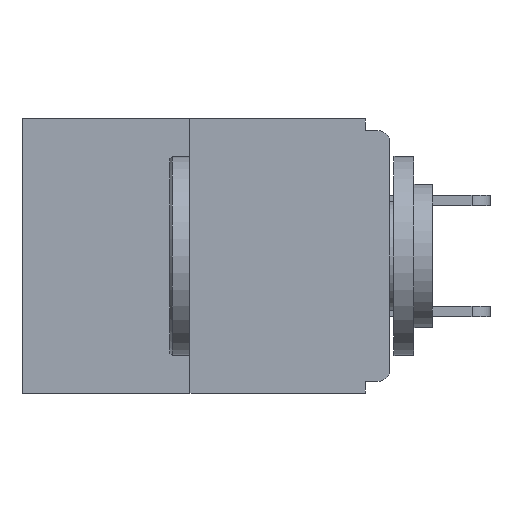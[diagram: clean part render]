
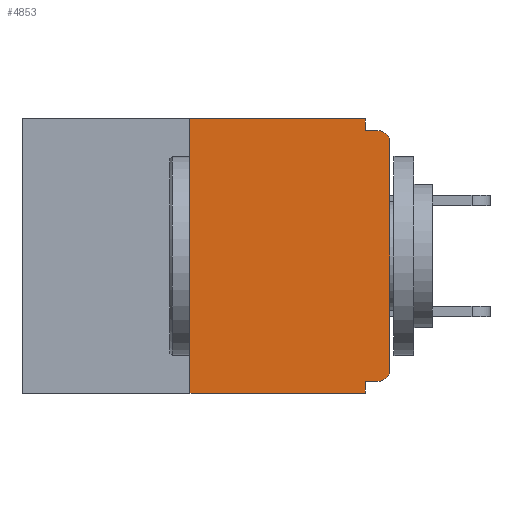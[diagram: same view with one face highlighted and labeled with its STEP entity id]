
A CAD part, left-side view. The second image highlights one B-rep face of the part: STEP entity #4853.
In plain terms, the highlighted planar face has unit normal (-1, 0, 0).
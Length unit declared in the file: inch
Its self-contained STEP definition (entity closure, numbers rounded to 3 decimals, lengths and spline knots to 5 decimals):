
#928 = CARTESIAN_POINT ( 'NONE',  ( 0., 0., -0.03 ) ) ;
#980 = DIRECTION ( 'NONE',  ( 0., 0., -1. ) ) ;
#1677 = VERTEX_POINT ( 'NONE', #18223 ) ;
#1706 = CARTESIAN_POINT ( 'NONE',  ( 0., 0., -0.328 ) ) ;
#1978 = CARTESIAN_POINT ( 'NONE',  ( 0., 0.031, -0.343 ) ) ;
#2062 = EDGE_CURVE ( 'NONE', #12273, #8762, #14587, .T. ) ;
#2663 = CARTESIAN_POINT ( 'NONE',  ( 0., 0.25, -0.343 ) ) ;
#2809 = EDGE_CURVE ( 'NONE', #20549, #18197, #7778, .T. ) ;
#2960 = DIRECTION ( 'NONE',  ( 1., 0., 0. ) ) ;
#3241 = ORIENTED_EDGE ( 'NONE', *, *, #2062, .T. ) ;
#3322 = VECTOR ( 'NONE', #9281, 39.37008 ) ;
#3625 = ORIENTED_EDGE ( 'NONE', *, *, #2809, .F. ) ;
#3954 = CARTESIAN_POINT ( 'NONE',  ( 0., 0.25, 0. ) ) ;
#4173 = EDGE_CURVE ( 'NONE', #14319, #5411, #5531, .T. ) ;
#4853 = ADVANCED_FACE ( 'NONE', ( #16636 ), #20152, .F. ) ;
#5059 = VECTOR ( 'NONE', #13648, 39.37008 ) ;
#5068 = CARTESIAN_POINT ( 'NONE',  ( 0., 0.46, 0. ) ) ;
#5254 = VECTOR ( 'NONE', #16502, 39.37008 ) ;
#5411 = VERTEX_POINT ( 'NONE', #1978 ) ;
#5472 = CARTESIAN_POINT ( 'NONE',  ( 0., 0.015, -0.313 ) ) ;
#5531 = LINE ( 'NONE', #12976, #7965 ) ;
#5664 = AXIS2_PLACEMENT_3D ( 'NONE', #13359, #6229, #980 ) ;
#6104 = LINE ( 'NONE', #17288, #19650 ) ;
#6229 = DIRECTION ( 'NONE',  ( -1., 0., 0. ) ) ;
#6690 = ORIENTED_EDGE ( 'NONE', *, *, #15009, .T. ) ;
#7367 = CARTESIAN_POINT ( 'NONE',  ( 0., 0.031, 0. ) ) ;
#7778 = LINE ( 'NONE', #5068, #5059 ) ;
#7844 = CARTESIAN_POINT ( 'NONE',  ( 0., 0., -0.313 ) ) ;
#7965 = VECTOR ( 'NONE', #18057, 39.37008 ) ;
#8101 = VERTEX_POINT ( 'NONE', #20424 ) ;
#8291 = CARTESIAN_POINT ( 'NONE',  ( 0., 0.031, 0. ) ) ;
#8558 = DIRECTION ( 'NONE',  ( 0., 0., 1. ) ) ;
#8621 = DIRECTION ( 'NONE',  ( 0., 1., 0. ) ) ;
#8762 = VERTEX_POINT ( 'NONE', #19467 ) ;
#9281 = DIRECTION ( 'NONE',  ( 0., -1., 0. ) ) ;
#10386 = LINE ( 'NONE', #1706, #16929 ) ;
#10979 = CARTESIAN_POINT ( 'NONE',  ( 0., 0., -0.015 ) ) ;
#11179 = DIRECTION ( 'NONE',  ( -1., 0., 0. ) ) ;
#12273 = VERTEX_POINT ( 'NONE', #928 ) ;
#12358 = VERTEX_POINT ( 'NONE', #7844 ) ;
#12701 = ORIENTED_EDGE ( 'NONE', *, *, #4173, .T. ) ;
#12844 = ORIENTED_EDGE ( 'NONE', *, *, #15701, .F. ) ;
#12976 = CARTESIAN_POINT ( 'NONE',  ( 0., 0.46, -0.343 ) ) ;
#13094 = EDGE_CURVE ( 'NONE', #18857, #8101, #10386, .T. ) ;
#13359 = CARTESIAN_POINT ( 'NONE',  ( 0., 0.015, -0.03 ) ) ;
#13399 = CARTESIAN_POINT ( 'NONE',  ( 0., 0.46, 0. ) ) ;
#13570 = EDGE_CURVE ( 'NONE', #18197, #1677, #18245, .T. ) ;
#13648 = DIRECTION ( 'NONE',  ( 0., -1., 0. ) ) ;
#14003 = CIRCLE ( 'NONE', #17605, 0.015 ) ;
#14144 = LINE ( 'NONE', #10979, #3322 ) ;
#14187 = VECTOR ( 'NONE', #20438, 39.37008 ) ;
#14319 = VERTEX_POINT ( 'NONE', #2663 ) ;
#14321 = ORIENTED_EDGE ( 'NONE', *, *, #13094, .F. ) ;
#14587 = CIRCLE ( 'NONE', #5664, 0.015 ) ;
#15009 = EDGE_CURVE ( 'NONE', #18857, #12358, #14003, .T. ) ;
#15413 = CARTESIAN_POINT ( 'NONE',  ( 0., 0.25, 0. ) ) ;
#15701 = EDGE_CURVE ( 'NONE', #8101, #5411, #6104, .T. ) ;
#15755 = EDGE_CURVE ( 'NONE', #14319, #20549, #19398, .T. ) ;
#16126 = ORIENTED_EDGE ( 'NONE', *, *, #13570, .F. ) ;
#16502 = DIRECTION ( 'NONE',  ( 0., 0., 1. ) ) ;
#16636 = FACE_OUTER_BOUND ( 'NONE', #21961, .T. ) ;
#16728 = DIRECTION ( 'NONE',  ( 0., 0., -1. ) ) ;
#16909 = ORIENTED_EDGE ( 'NONE', *, *, #21146, .F. ) ;
#16929 = VECTOR ( 'NONE', #8621, 39.37008 ) ;
#17288 = CARTESIAN_POINT ( 'NONE',  ( 0., 0.031, -0.343 ) ) ;
#17605 = AXIS2_PLACEMENT_3D ( 'NONE', #5472, #11179, #21613 ) ;
#17744 = VECTOR ( 'NONE', #8558, 39.37008 ) ;
#18057 = DIRECTION ( 'NONE',  ( 0., -1., 0. ) ) ;
#18197 = VERTEX_POINT ( 'NONE', #7367 ) ;
#18223 = CARTESIAN_POINT ( 'NONE',  ( 0., 0.031, -0.015 ) ) ;
#18245 = LINE ( 'NONE', #8291, #14187 ) ;
#18857 = VERTEX_POINT ( 'NONE', #19244 ) ;
#18964 = DIRECTION ( 'NONE',  ( 0., 0., -1. ) ) ;
#19094 = ORIENTED_EDGE ( 'NONE', *, *, #20122, .T. ) ;
#19244 = CARTESIAN_POINT ( 'NONE',  ( 0., 0.015, -0.328 ) ) ;
#19398 = LINE ( 'NONE', #15413, #17744 ) ;
#19467 = CARTESIAN_POINT ( 'NONE',  ( 0., 0.015, -0.015 ) ) ;
#19650 = VECTOR ( 'NONE', #18964, 39.37008 ) ;
#20122 = EDGE_CURVE ( 'NONE', #12358, #12273, #20968, .T. ) ;
#20152 = PLANE ( 'NONE',  #22276 ) ;
#20424 = CARTESIAN_POINT ( 'NONE',  ( 0., 0.031, -0.328 ) ) ;
#20438 = DIRECTION ( 'NONE',  ( 0., 0., -1. ) ) ;
#20549 = VERTEX_POINT ( 'NONE', #3954 ) ;
#20968 = LINE ( 'NONE', #21793, #5254 ) ;
#21146 = EDGE_CURVE ( 'NONE', #1677, #8762, #14144, .T. ) ;
#21461 = ORIENTED_EDGE ( 'NONE', *, *, #15755, .F. ) ;
#21613 = DIRECTION ( 'NONE',  ( 0., 0., -1. ) ) ;
#21793 = CARTESIAN_POINT ( 'NONE',  ( 0., 0., 0. ) ) ;
#21961 = EDGE_LOOP ( 'NONE', ( #3625, #21461, #12701, #12844, #14321, #6690, #19094, #3241, #16909, #16126 ) ) ;
#22276 = AXIS2_PLACEMENT_3D ( 'NONE', #13399, #2960, #16728 ) ;
